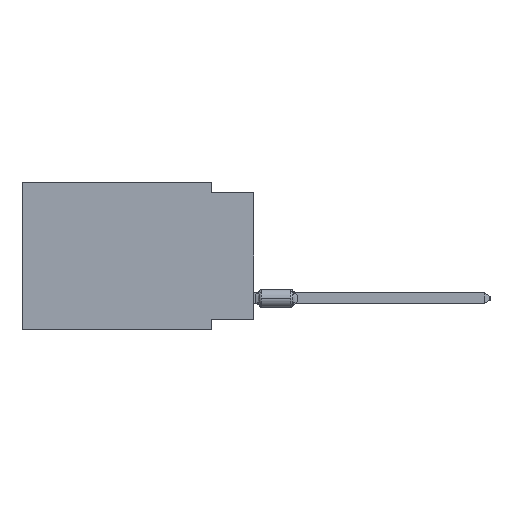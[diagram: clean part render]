
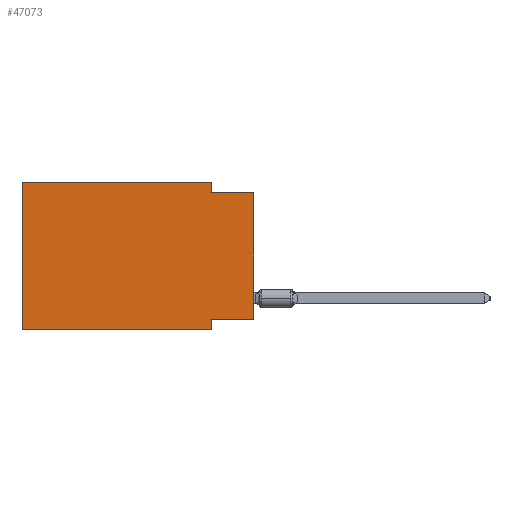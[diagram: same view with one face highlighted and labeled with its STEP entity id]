
A CAD part, left-side view. The second image highlights one B-rep face of the part: STEP entity #47073.
In plain terms, the highlighted planar face has unit normal (-1, 0, 0).
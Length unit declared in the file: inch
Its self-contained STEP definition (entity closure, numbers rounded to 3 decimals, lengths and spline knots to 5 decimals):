
#160 = EDGE_CURVE ( 'NONE', #61006, #51932, #63025, .T. ) ;
#1467 = CARTESIAN_POINT ( 'NONE',  ( 0., 0.1, -0.35 ) ) ;
#2463 = VECTOR ( 'NONE', #59679, 39.37008 ) ;
#3972 = LINE ( 'NONE', #84676, #57223 ) ;
#4178 = DIRECTION ( 'NONE',  ( 1., 0., 0. ) ) ;
#6501 = CARTESIAN_POINT ( 'NONE',  ( 0., 0.55, -0.35 ) ) ;
#8052 = ORIENTED_EDGE ( 'NONE', *, *, #73049, .F. ) ;
#10160 = CARTESIAN_POINT ( 'NONE',  ( 0., 0., -0.025 ) ) ;
#11333 = ORIENTED_EDGE ( 'NONE', *, *, #12621, .F. ) ;
#11669 = CARTESIAN_POINT ( 'NONE',  ( 0., 0.55, 0. ) ) ;
#12001 = ORIENTED_EDGE ( 'NONE', *, *, #24894, .T. ) ;
#12621 = EDGE_CURVE ( 'NONE', #76407, #83919, #27800, .T. ) ;
#16770 = CARTESIAN_POINT ( 'NONE',  ( 0., 0.55, 0. ) ) ;
#18803 = LINE ( 'NONE', #27351, #59758 ) ;
#20562 = EDGE_CURVE ( 'NONE', #44661, #60480, #23549, .T. ) ;
#21973 = CARTESIAN_POINT ( 'NONE',  ( 0., 0., -0.325 ) ) ;
#23549 = LINE ( 'NONE', #21973, #40334 ) ;
#24570 = ORIENTED_EDGE ( 'NONE', *, *, #98434, .F. ) ;
#24894 = EDGE_CURVE ( 'NONE', #44661, #79329, #18803, .T. ) ;
#26970 = DIRECTION ( 'NONE',  ( 0., -1., 0. ) ) ;
#27351 = CARTESIAN_POINT ( 'NONE',  ( 0., 0., 0. ) ) ;
#27800 = LINE ( 'NONE', #52865, #100360 ) ;
#28593 = CARTESIAN_POINT ( 'NONE',  ( 0., 0., -0.025 ) ) ;
#28749 = FACE_OUTER_BOUND ( 'NONE', #88075, .T. ) ;
#28865 = DIRECTION ( 'NONE',  ( 0., -1., 0. ) ) ;
#28893 = ORIENTED_EDGE ( 'NONE', *, *, #20562, .F. ) ;
#33535 = LINE ( 'NONE', #1467, #2463 ) ;
#36173 = VERTEX_POINT ( 'NONE', #49405 ) ;
#37072 = CARTESIAN_POINT ( 'NONE',  ( 0., 0.1, 0. ) ) ;
#37527 = VECTOR ( 'NONE', #28865, 39.37008 ) ;
#39061 = CARTESIAN_POINT ( 'NONE',  ( 0., 0., -0.325 ) ) ;
#40334 = VECTOR ( 'NONE', #95166, 39.37008 ) ;
#40960 = CARTESIAN_POINT ( 'NONE',  ( 0., 0.1, -0.325 ) ) ;
#40964 = CARTESIAN_POINT ( 'NONE',  ( 0., 0.1, -0.35 ) ) ;
#43274 = LINE ( 'NONE', #10160, #48844 ) ;
#43393 = ORIENTED_EDGE ( 'NONE', *, *, #93432, .F. ) ;
#44661 = VERTEX_POINT ( 'NONE', #39061 ) ;
#47073 = ADVANCED_FACE ( 'NONE', ( #28749 ), #90919, .F. ) ;
#48844 = VECTOR ( 'NONE', #59810, 39.37008 ) ;
#49160 = ORIENTED_EDGE ( 'NONE', *, *, #92738, .F. ) ;
#49335 = DIRECTION ( 'NONE',  ( 0., 0., 1. ) ) ;
#49405 = CARTESIAN_POINT ( 'NONE',  ( 0., 0.55, 0. ) ) ;
#51932 = VERTEX_POINT ( 'NONE', #40964 ) ;
#52865 = CARTESIAN_POINT ( 'NONE',  ( 0., 0.1, 0. ) ) ;
#57223 = VECTOR ( 'NONE', #26970, 39.37008 ) ;
#57355 = CARTESIAN_POINT ( 'NONE',  ( 0., 0.1, -0.025 ) ) ;
#59679 = DIRECTION ( 'NONE',  ( 0., 0., -1. ) ) ;
#59758 = VECTOR ( 'NONE', #59911, 39.37008 ) ;
#59810 = DIRECTION ( 'NONE',  ( 0., -1., 0. ) ) ;
#59911 = DIRECTION ( 'NONE',  ( 0., 0., 1. ) ) ;
#60270 = DIRECTION ( 'NONE',  ( 0., 0., -1. ) ) ;
#60364 = DIRECTION ( 'NONE',  ( 0., 0., -1. ) ) ;
#60480 = VERTEX_POINT ( 'NONE', #40960 ) ;
#61006 = VERTEX_POINT ( 'NONE', #6501 ) ;
#63025 = LINE ( 'NONE', #95114, #37527 ) ;
#66248 = AXIS2_PLACEMENT_3D ( 'NONE', #11669, #4178, #60270 ) ;
#70166 = VECTOR ( 'NONE', #49335, 39.37008 ) ;
#73049 = EDGE_CURVE ( 'NONE', #83919, #79329, #43274, .T. ) ;
#76407 = VERTEX_POINT ( 'NONE', #37072 ) ;
#79329 = VERTEX_POINT ( 'NONE', #28593 ) ;
#83919 = VERTEX_POINT ( 'NONE', #57355 ) ;
#84676 = CARTESIAN_POINT ( 'NONE',  ( 0., 0.55, 0. ) ) ;
#88075 = EDGE_LOOP ( 'NONE', ( #12001, #8052, #11333, #49160, #24570, #97792, #43393, #28893 ) ) ;
#90919 = PLANE ( 'NONE',  #66248 ) ;
#92738 = EDGE_CURVE ( 'NONE', #36173, #76407, #3972, .T. ) ;
#93432 = EDGE_CURVE ( 'NONE', #60480, #51932, #33535, .T. ) ;
#95114 = CARTESIAN_POINT ( 'NONE',  ( 0., 0.55, -0.35 ) ) ;
#95166 = DIRECTION ( 'NONE',  ( 0., 1., 0. ) ) ;
#97792 = ORIENTED_EDGE ( 'NONE', *, *, #160, .T. ) ;
#98434 = EDGE_CURVE ( 'NONE', #61006, #36173, #99573, .T. ) ;
#99573 = LINE ( 'NONE', #16770, #70166 ) ;
#100360 = VECTOR ( 'NONE', #60364, 39.37008 ) ;
